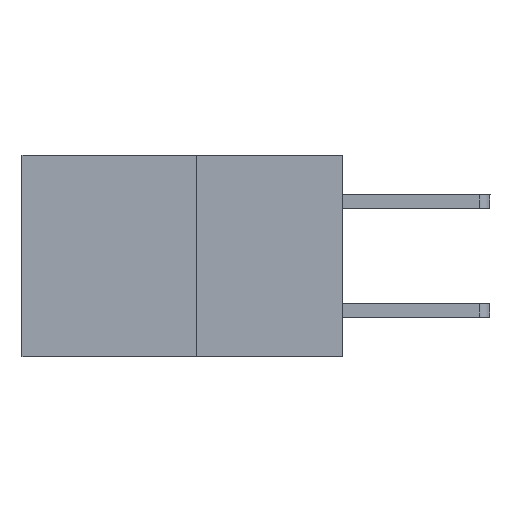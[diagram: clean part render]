
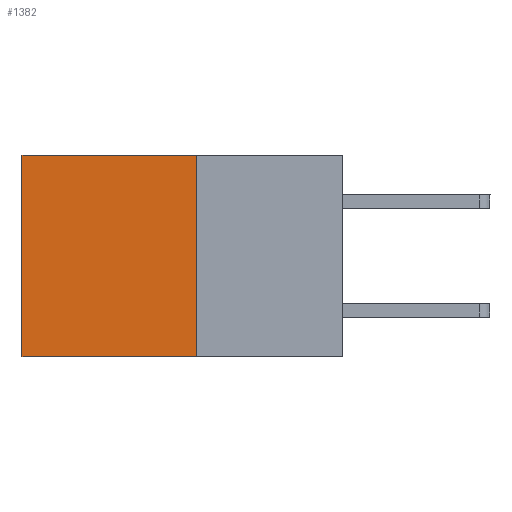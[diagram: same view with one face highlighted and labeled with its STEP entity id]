
A CAD part, left-side view. The second image highlights one B-rep face of the part: STEP entity #1382.
In plain terms, the highlighted planar face has unit normal (-1, 0, 0).
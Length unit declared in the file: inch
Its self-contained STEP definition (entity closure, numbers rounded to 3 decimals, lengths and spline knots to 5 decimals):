
#528 = VECTOR ( 'NONE', #6598, 39.37008 ) ;
#576 = CARTESIAN_POINT ( 'NONE',  ( 0.277, 0.27, 0. ) ) ;
#1107 = VERTEX_POINT ( 'NONE', #10410 ) ;
#1305 = CARTESIAN_POINT ( 'NONE',  ( 0.277, 0.27, -0.37 ) ) ;
#1382 = ADVANCED_FACE ( 'NONE', ( #1530 ), #11806, .F. ) ;
#1530 = FACE_OUTER_BOUND ( 'NONE', #6655, .T. ) ;
#2566 = DIRECTION ( 'NONE',  ( 1., 0., 0. ) ) ;
#2923 = LINE ( 'NONE', #4887, #528 ) ;
#2974 = VECTOR ( 'NONE', #10928, 39.37008 ) ;
#2986 = ORIENTED_EDGE ( 'NONE', *, *, #3470, .F. ) ;
#3470 = EDGE_CURVE ( 'NONE', #6713, #8507, #5222, .T. ) ;
#3519 = CARTESIAN_POINT ( 'NONE',  ( 0.277, 0.27, -0.37 ) ) ;
#4265 = CARTESIAN_POINT ( 'NONE',  ( 0.277, 0.27, -0.37 ) ) ;
#4287 = ORIENTED_EDGE ( 'NONE', *, *, #9733, .F. ) ;
#4352 = CARTESIAN_POINT ( 'NONE',  ( 0.277, 0.27, -0.37 ) ) ;
#4887 = CARTESIAN_POINT ( 'NONE',  ( 0.277, 0.27, 0. ) ) ;
#4920 = EDGE_CURVE ( 'NONE', #10277, #1107, #2923, .T. ) ;
#4958 = LINE ( 'NONE', #7882, #8070 ) ;
#5222 = LINE ( 'NONE', #4265, #6813 ) ;
#5809 = DIRECTION ( 'NONE',  ( 0., 0., -1. ) ) ;
#6598 = DIRECTION ( 'NONE',  ( 0., 1., 0. ) ) ;
#6655 = EDGE_LOOP ( 'NONE', ( #7204, #2986, #4287, #11377 ) ) ;
#6713 = VERTEX_POINT ( 'NONE', #1305 ) ;
#6813 = VECTOR ( 'NONE', #8895, 39.37008 ) ;
#7204 = ORIENTED_EDGE ( 'NONE', *, *, #11797, .T. ) ;
#7882 = CARTESIAN_POINT ( 'NONE',  ( 0.277, 0.59, -0.37 ) ) ;
#8070 = VECTOR ( 'NONE', #5809, 39.37008 ) ;
#8143 = CARTESIAN_POINT ( 'NONE',  ( 0.277, 0.59, -0.37 ) ) ;
#8507 = VERTEX_POINT ( 'NONE', #8143 ) ;
#8577 = AXIS2_PLACEMENT_3D ( 'NONE', #4352, #2566, #10896 ) ;
#8895 = DIRECTION ( 'NONE',  ( 0., 1., 0. ) ) ;
#9202 = LINE ( 'NONE', #3519, #2974 ) ;
#9733 = EDGE_CURVE ( 'NONE', #10277, #6713, #9202, .T. ) ;
#10277 = VERTEX_POINT ( 'NONE', #576 ) ;
#10410 = CARTESIAN_POINT ( 'NONE',  ( 0.277, 0.59, 0. ) ) ;
#10896 = DIRECTION ( 'NONE',  ( 0., 0., -1. ) ) ;
#10928 = DIRECTION ( 'NONE',  ( 0., 0., -1. ) ) ;
#11377 = ORIENTED_EDGE ( 'NONE', *, *, #4920, .T. ) ;
#11797 = EDGE_CURVE ( 'NONE', #1107, #8507, #4958, .T. ) ;
#11806 = PLANE ( 'NONE',  #8577 ) ;
